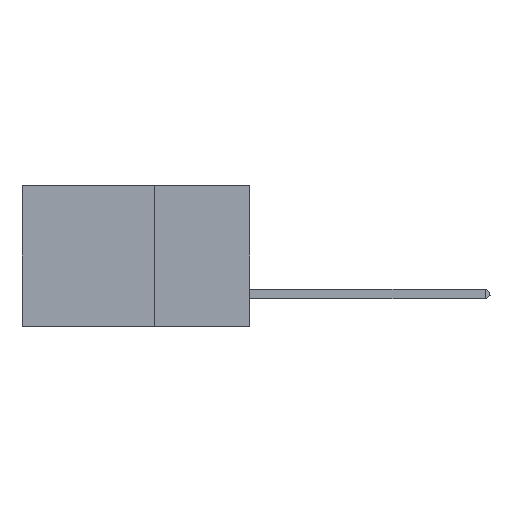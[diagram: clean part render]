
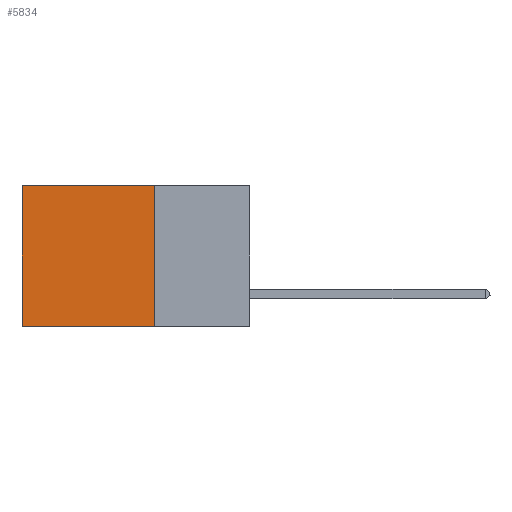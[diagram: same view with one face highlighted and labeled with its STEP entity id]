
A CAD part, left-side view. The second image highlights one B-rep face of the part: STEP entity #5834.
In plain terms, the highlighted planar face has unit normal (-1, 0, 0).
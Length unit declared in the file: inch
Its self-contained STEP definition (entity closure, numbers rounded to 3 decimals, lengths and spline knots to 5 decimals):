
#201 = CARTESIAN_POINT ( 'NONE',  ( 0.2875, 0.6, 0. ) ) ;
#768 = ORIENTED_EDGE ( 'NONE', *, *, #11155, .T. ) ;
#1240 = EDGE_CURVE ( 'NONE', #1936, #19082, #18136, .T. ) ;
#1540 = DIRECTION ( 'NONE',  ( 0., 1., 0. ) ) ;
#1936 = VERTEX_POINT ( 'NONE', #11915 ) ;
#2029 = LINE ( 'NONE', #201, #7355 ) ;
#3488 = ORIENTED_EDGE ( 'NONE', *, *, #11611, .F. ) ;
#3798 = DIRECTION ( 'NONE',  ( 0., 0., -1. ) ) ;
#4185 = AXIS2_PLACEMENT_3D ( 'NONE', #15827, #10063, #3798 ) ;
#4920 = EDGE_LOOP ( 'NONE', ( #14503, #3488, #7663, #768 ) ) ;
#4955 = EDGE_CURVE ( 'NONE', #9489, #17452, #2029, .T. ) ;
#5009 = VECTOR ( 'NONE', #9354, 39.37008 ) ;
#5322 = VECTOR ( 'NONE', #10321, 39.37008 ) ;
#5834 = ADVANCED_FACE ( 'NONE', ( #16186 ), #7568, .F. ) ;
#5929 = CARTESIAN_POINT ( 'NONE',  ( 0.2875, 0.25, 0. ) ) ;
#7355 = VECTOR ( 'NONE', #13558, 39.37008 ) ;
#7493 = CARTESIAN_POINT ( 'NONE',  ( 0.2875, 0.25, -0.37 ) ) ;
#7568 = PLANE ( 'NONE',  #4185 ) ;
#7663 = ORIENTED_EDGE ( 'NONE', *, *, #1240, .F. ) ;
#8723 = LINE ( 'NONE', #7493, #15956 ) ;
#9354 = DIRECTION ( 'NONE',  ( 0., 1., 0. ) ) ;
#9489 = VERTEX_POINT ( 'NONE', #16365 ) ;
#10063 = DIRECTION ( 'NONE',  ( 1., 0., 0. ) ) ;
#10321 = DIRECTION ( 'NONE',  ( 0., 0., -1. ) ) ;
#11155 = EDGE_CURVE ( 'NONE', #1936, #9489, #16446, .T. ) ;
#11611 = EDGE_CURVE ( 'NONE', #19082, #17452, #8723, .T. ) ;
#11915 = CARTESIAN_POINT ( 'NONE',  ( 0.2875, 0.25, 0. ) ) ;
#12274 = CARTESIAN_POINT ( 'NONE',  ( 0.2875, 0.25, 0. ) ) ;
#13558 = DIRECTION ( 'NONE',  ( 0., 0., -1. ) ) ;
#14503 = ORIENTED_EDGE ( 'NONE', *, *, #4955, .T. ) ;
#15827 = CARTESIAN_POINT ( 'NONE',  ( 0.2875, 0.25, 0. ) ) ;
#15956 = VECTOR ( 'NONE', #1540, 39.37008 ) ;
#16186 = FACE_OUTER_BOUND ( 'NONE', #4920, .T. ) ;
#16365 = CARTESIAN_POINT ( 'NONE',  ( 0.2875, 0.6, 0. ) ) ;
#16446 = LINE ( 'NONE', #12274, #5009 ) ;
#17237 = CARTESIAN_POINT ( 'NONE',  ( 0.2875, 0.6, -0.37 ) ) ;
#17452 = VERTEX_POINT ( 'NONE', #17237 ) ;
#18008 = CARTESIAN_POINT ( 'NONE',  ( 0.2875, 0.25, -0.37 ) ) ;
#18136 = LINE ( 'NONE', #5929, #5322 ) ;
#19082 = VERTEX_POINT ( 'NONE', #18008 ) ;
